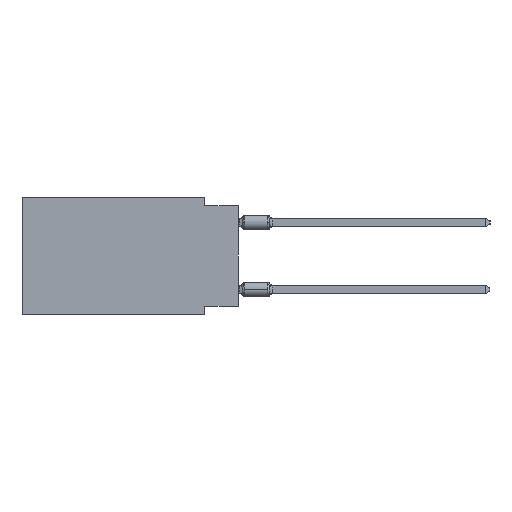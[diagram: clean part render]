
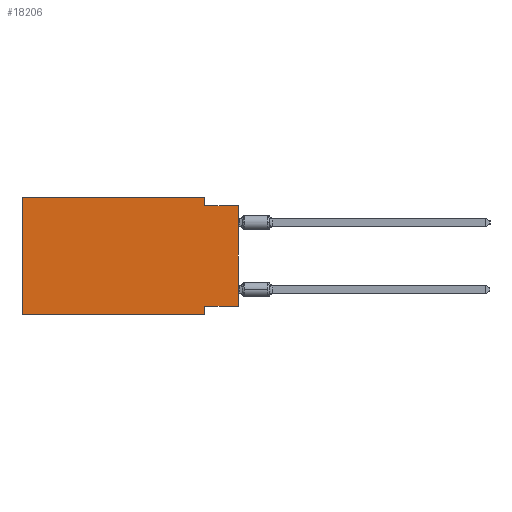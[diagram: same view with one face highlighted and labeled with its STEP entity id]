
A CAD part, left-side view. The second image highlights one B-rep face of the part: STEP entity #18206.
In plain terms, the highlighted planar face has unit normal (-1, 0, 0).
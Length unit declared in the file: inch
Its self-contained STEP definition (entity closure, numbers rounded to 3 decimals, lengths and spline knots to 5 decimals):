
#26 = DIRECTION ( 'NONE',  ( 0., -1., 0. ) ) ;
#58 = EDGE_CURVE ( 'NONE', #19827, #34686, #31884, .T. ) ;
#88 = AXIS2_PLACEMENT_3D ( 'NONE', #13152, #17785, #10477 ) ;
#1017 = VERTEX_POINT ( 'NONE', #42812 ) ;
#1808 = CARTESIAN_POINT ( 'NONE',  ( 0., 0.1, -0.025 ) ) ;
#2551 = VERTEX_POINT ( 'NONE', #1808 ) ;
#2814 = EDGE_CURVE ( 'NONE', #19827, #7420, #11786, .T. ) ;
#3667 = DIRECTION ( 'NONE',  ( 0., 0., -1. ) ) ;
#4353 = EDGE_CURVE ( 'NONE', #34686, #1017, #30162, .T. ) ;
#5449 = VERTEX_POINT ( 'NONE', #8696 ) ;
#5590 = VECTOR ( 'NONE', #12865, 39.37008 ) ;
#6115 = EDGE_CURVE ( 'NONE', #1017, #2551, #29864, .T. ) ;
#6985 = VECTOR ( 'NONE', #26, 39.37008 ) ;
#7420 = VERTEX_POINT ( 'NONE', #34350 ) ;
#8696 = CARTESIAN_POINT ( 'NONE',  ( 0., 0., -0.325 ) ) ;
#8970 = LINE ( 'NONE', #42722, #5590 ) ;
#10317 = CARTESIAN_POINT ( 'NONE',  ( 0., 0.1, 0. ) ) ;
#10477 = DIRECTION ( 'NONE',  ( 0., 0., -1. ) ) ;
#11332 = DIRECTION ( 'NONE',  ( 0., -1., 0. ) ) ;
#11786 = LINE ( 'NONE', #37734, #43725 ) ;
#12865 = DIRECTION ( 'NONE',  ( 0., 0., -1. ) ) ;
#13152 = CARTESIAN_POINT ( 'NONE',  ( 0., 0.645, 0. ) ) ;
#13326 = CARTESIAN_POINT ( 'NONE',  ( 0., 0., -0.025 ) ) ;
#13638 = FACE_OUTER_BOUND ( 'NONE', #28141, .T. ) ;
#15234 = CARTESIAN_POINT ( 'NONE',  ( 0., 0.645, 0. ) ) ;
#15776 = ORIENTED_EDGE ( 'NONE', *, *, #20617, .T. ) ;
#17785 = DIRECTION ( 'NONE',  ( 1., 0., 0. ) ) ;
#18206 = ADVANCED_FACE ( 'NONE', ( #13638 ), #44003, .F. ) ;
#18706 = EDGE_CURVE ( 'NONE', #30625, #7420, #8970, .T. ) ;
#19424 = VECTOR ( 'NONE', #32830, 39.37008 ) ;
#19827 = VERTEX_POINT ( 'NONE', #30504 ) ;
#19951 = ORIENTED_EDGE ( 'NONE', *, *, #27744, .F. ) ;
#20397 = ORIENTED_EDGE ( 'NONE', *, *, #58, .F. ) ;
#20617 = EDGE_CURVE ( 'NONE', #5449, #23351, #20662, .T. ) ;
#20662 = LINE ( 'NONE', #28229, #42404 ) ;
#23351 = VERTEX_POINT ( 'NONE', #13326 ) ;
#25730 = CARTESIAN_POINT ( 'NONE',  ( 0., 0., -0.325 ) ) ;
#25950 = VECTOR ( 'NONE', #3667, 39.37008 ) ;
#27040 = DIRECTION ( 'NONE',  ( 0., 0., 1. ) ) ;
#27692 = EDGE_CURVE ( 'NONE', #2551, #23351, #36748, .T. ) ;
#27744 = EDGE_CURVE ( 'NONE', #5449, #30625, #36273, .T. ) ;
#28141 = EDGE_LOOP ( 'NONE', ( #15776, #45876, #35131, #30011, #20397, #33103, #45865, #19951 ) ) ;
#28229 = CARTESIAN_POINT ( 'NONE',  ( 0., 0., 0. ) ) ;
#29864 = LINE ( 'NONE', #10317, #25950 ) ;
#30011 = ORIENTED_EDGE ( 'NONE', *, *, #4353, .F. ) ;
#30162 = LINE ( 'NONE', #15234, #32847 ) ;
#30359 = VECTOR ( 'NONE', #27040, 39.37008 ) ;
#30504 = CARTESIAN_POINT ( 'NONE',  ( 0., 0.645, -0.35 ) ) ;
#30625 = VERTEX_POINT ( 'NONE', #43791 ) ;
#31884 = LINE ( 'NONE', #46140, #30359 ) ;
#32830 = DIRECTION ( 'NONE',  ( 0., 1., 0. ) ) ;
#32847 = VECTOR ( 'NONE', #11332, 39.37008 ) ;
#33073 = CARTESIAN_POINT ( 'NONE',  ( 0., 0., -0.025 ) ) ;
#33103 = ORIENTED_EDGE ( 'NONE', *, *, #2814, .T. ) ;
#34350 = CARTESIAN_POINT ( 'NONE',  ( 0., 0.1, -0.35 ) ) ;
#34686 = VERTEX_POINT ( 'NONE', #44446 ) ;
#35131 = ORIENTED_EDGE ( 'NONE', *, *, #6115, .F. ) ;
#36273 = LINE ( 'NONE', #25730, #19424 ) ;
#36748 = LINE ( 'NONE', #33073, #6985 ) ;
#37734 = CARTESIAN_POINT ( 'NONE',  ( 0., 0.645, -0.35 ) ) ;
#39469 = DIRECTION ( 'NONE',  ( 0., 0., 1. ) ) ;
#41658 = DIRECTION ( 'NONE',  ( 0., -1., 0. ) ) ;
#42404 = VECTOR ( 'NONE', #39469, 39.37008 ) ;
#42722 = CARTESIAN_POINT ( 'NONE',  ( 0., 0.1, -0.35 ) ) ;
#42812 = CARTESIAN_POINT ( 'NONE',  ( 0., 0.1, 0. ) ) ;
#43725 = VECTOR ( 'NONE', #41658, 39.37008 ) ;
#43791 = CARTESIAN_POINT ( 'NONE',  ( 0., 0.1, -0.325 ) ) ;
#44003 = PLANE ( 'NONE',  #88 ) ;
#44446 = CARTESIAN_POINT ( 'NONE',  ( 0., 0.645, 0. ) ) ;
#45865 = ORIENTED_EDGE ( 'NONE', *, *, #18706, .F. ) ;
#45876 = ORIENTED_EDGE ( 'NONE', *, *, #27692, .F. ) ;
#46140 = CARTESIAN_POINT ( 'NONE',  ( 0., 0.645, 0. ) ) ;
